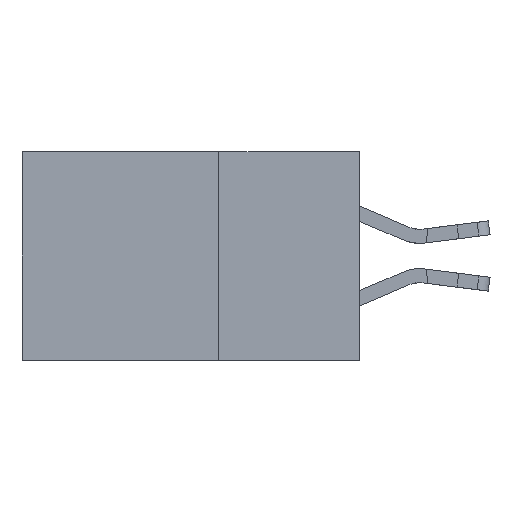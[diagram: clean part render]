
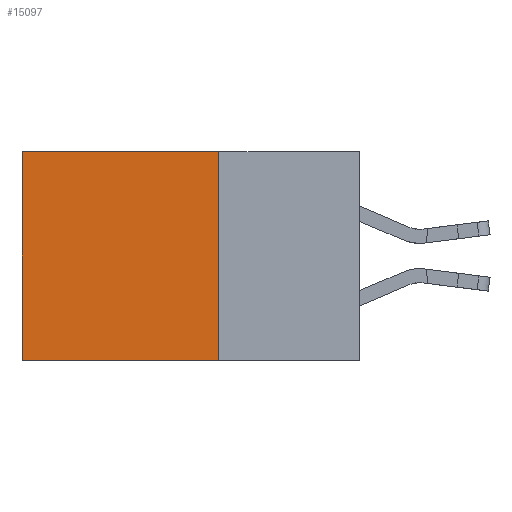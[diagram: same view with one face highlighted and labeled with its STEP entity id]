
A CAD part, left-side view. The second image highlights one B-rep face of the part: STEP entity #15097.
In plain terms, the highlighted planar face has unit normal (-1, 0, 0).
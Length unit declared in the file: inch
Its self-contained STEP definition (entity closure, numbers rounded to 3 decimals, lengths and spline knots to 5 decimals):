
#1236 = CARTESIAN_POINT ( 'NONE',  ( 0.2875, 0.25, 0. ) ) ;
#2481 = VECTOR ( 'NONE', #7840, 39.37008 ) ;
#4034 = DIRECTION ( 'NONE',  ( 0., 0., -1. ) ) ;
#4503 = ORIENTED_EDGE ( 'NONE', *, *, #14497, .F. ) ;
#7041 = FACE_OUTER_BOUND ( 'NONE', #32969, .T. ) ;
#7455 = LINE ( 'NONE', #20283, #12173 ) ;
#7840 = DIRECTION ( 'NONE',  ( 0., 1., 0. ) ) ;
#9177 = CARTESIAN_POINT ( 'NONE',  ( 0.2875, 0.25, 0. ) ) ;
#10352 = ORIENTED_EDGE ( 'NONE', *, *, #21025, .T. ) ;
#11554 = AXIS2_PLACEMENT_3D ( 'NONE', #1236, #15171, #4034 ) ;
#12173 = VECTOR ( 'NONE', #20405, 39.37008 ) ;
#12266 = PLANE ( 'NONE',  #11554 ) ;
#12951 = VERTEX_POINT ( 'NONE', #21731 ) ;
#13879 = VERTEX_POINT ( 'NONE', #20088 ) ;
#14494 = DIRECTION ( 'NONE',  ( 0., 0., -1. ) ) ;
#14497 = EDGE_CURVE ( 'NONE', #13879, #35262, #7455, .T. ) ;
#15097 = ADVANCED_FACE ( 'NONE', ( #7041 ), #12266, .F. ) ;
#15171 = DIRECTION ( 'NONE',  ( 1., 0., 0. ) ) ;
#16047 = LINE ( 'NONE', #9177, #23389 ) ;
#17412 = ORIENTED_EDGE ( 'NONE', *, *, #27274, .F. ) ;
#18650 = CARTESIAN_POINT ( 'NONE',  ( 0.2875, 0.25, 0. ) ) ;
#19036 = LINE ( 'NONE', #18650, #2481 ) ;
#20088 = CARTESIAN_POINT ( 'NONE',  ( 0.2875, 0.25, -0.37 ) ) ;
#20283 = CARTESIAN_POINT ( 'NONE',  ( 0.2875, 0.25, -0.37 ) ) ;
#20405 = DIRECTION ( 'NONE',  ( 0., 1., 0. ) ) ;
#21025 = EDGE_CURVE ( 'NONE', #12951, #21347, #19036, .T. ) ;
#21347 = VERTEX_POINT ( 'NONE', #27829 ) ;
#21731 = CARTESIAN_POINT ( 'NONE',  ( 0.2875, 0.25, 0. ) ) ;
#23389 = VECTOR ( 'NONE', #14494, 39.37008 ) ;
#25883 = LINE ( 'NONE', #32132, #32362 ) ;
#27274 = EDGE_CURVE ( 'NONE', #12951, #13879, #16047, .T. ) ;
#27829 = CARTESIAN_POINT ( 'NONE',  ( 0.2875, 0.6, 0. ) ) ;
#29551 = EDGE_CURVE ( 'NONE', #21347, #35262, #25883, .T. ) ;
#31880 = DIRECTION ( 'NONE',  ( 0., 0., -1. ) ) ;
#32132 = CARTESIAN_POINT ( 'NONE',  ( 0.2875, 0.6, 0. ) ) ;
#32362 = VECTOR ( 'NONE', #31880, 39.37008 ) ;
#32756 = ORIENTED_EDGE ( 'NONE', *, *, #29551, .T. ) ;
#32969 = EDGE_LOOP ( 'NONE', ( #32756, #4503, #17412, #10352 ) ) ;
#34014 = CARTESIAN_POINT ( 'NONE',  ( 0.2875, 0.6, -0.37 ) ) ;
#35262 = VERTEX_POINT ( 'NONE', #34014 ) ;
